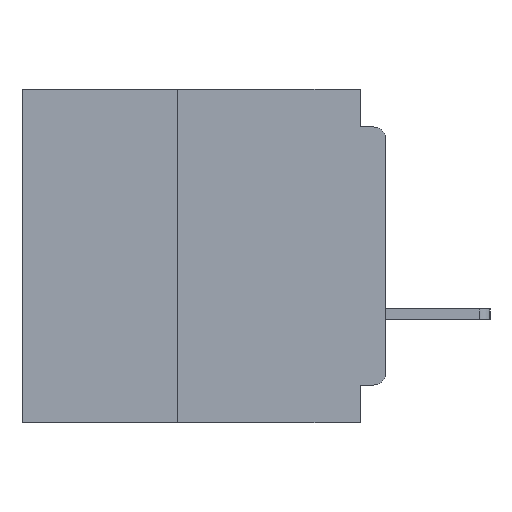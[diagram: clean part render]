
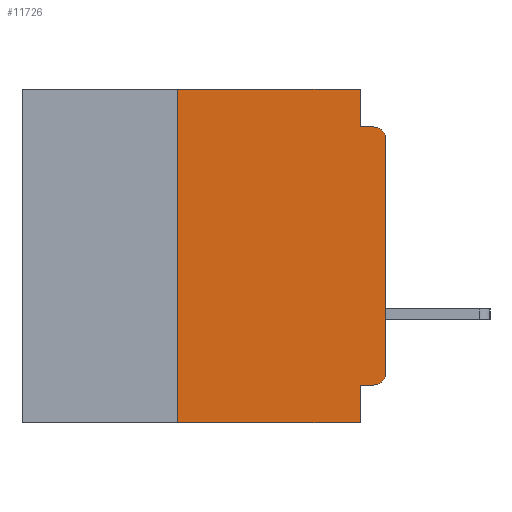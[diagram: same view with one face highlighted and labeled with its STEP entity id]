
A CAD part, left-side view. The second image highlights one B-rep face of the part: STEP entity #11726.
In plain terms, the highlighted planar face has unit normal (-1, 0, 0).
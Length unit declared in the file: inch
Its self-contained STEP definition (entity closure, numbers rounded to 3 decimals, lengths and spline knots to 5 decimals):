
#1133 = EDGE_CURVE ( 'NONE', #33137, #47126, #41011, .T. ) ;
#1188 = VECTOR ( 'NONE', #29116, 39.37008 ) ;
#1340 = CIRCLE ( 'NONE', #21619, 0.015 ) ;
#1385 = ORIENTED_EDGE ( 'NONE', *, *, #33223, .T. ) ;
#3551 = EDGE_CURVE ( 'NONE', #46628, #23718, #9136, .T. ) ;
#3782 = EDGE_CURVE ( 'NONE', #47126, #16703, #18458, .T. ) ;
#3885 = PLANE ( 'NONE',  #14189 ) ;
#4304 = LINE ( 'NONE', #25368, #42964 ) ;
#5230 = EDGE_CURVE ( 'NONE', #31758, #46628, #37131, .T. ) ;
#6052 = LINE ( 'NONE', #44029, #17165 ) ;
#7671 = CARTESIAN_POINT ( 'NONE',  ( 0., 0.437, 0. ) ) ;
#8571 = ORIENTED_EDGE ( 'NONE', *, *, #3782, .F. ) ;
#8986 = FACE_OUTER_BOUND ( 'NONE', #24166, .T. ) ;
#9136 = LINE ( 'NONE', #38466, #37839 ) ;
#11415 = DIRECTION ( 'NONE',  ( 0., 0., -1. ) ) ;
#11451 = ORIENTED_EDGE ( 'NONE', *, *, #3551, .F. ) ;
#11491 = CARTESIAN_POINT ( 'NONE',  ( 0., 0.25, 0. ) ) ;
#11572 = EDGE_CURVE ( 'NONE', #14571, #30251, #6052, .T. ) ;
#11726 = ADVANCED_FACE ( 'NONE', ( #8986 ), #3885, .F. ) ;
#13994 = CARTESIAN_POINT ( 'NONE',  ( 0., 0.015, -0.355 ) ) ;
#14189 = AXIS2_PLACEMENT_3D ( 'NONE', #7671, #33876, #11415 ) ;
#14262 = EDGE_CURVE ( 'NONE', #33137, #14571, #38580, .T. ) ;
#14571 = VERTEX_POINT ( 'NONE', #34019 ) ;
#16144 = DIRECTION ( 'NONE',  ( -1., 0., 0. ) ) ;
#16207 = VECTOR ( 'NONE', #44451, 39.37008 ) ;
#16296 = ORIENTED_EDGE ( 'NONE', *, *, #5230, .F. ) ;
#16703 = VERTEX_POINT ( 'NONE', #31825 ) ;
#17165 = VECTOR ( 'NONE', #32747, 39.37008 ) ;
#17273 = VECTOR ( 'NONE', #23125, 39.37008 ) ;
#18458 = LINE ( 'NONE', #23476, #17273 ) ;
#19808 = ORIENTED_EDGE ( 'NONE', *, *, #29904, .F. ) ;
#19829 = LINE ( 'NONE', #27886, #38569 ) ;
#21082 = CARTESIAN_POINT ( 'NONE',  ( 0., 0.015, -0.34 ) ) ;
#21416 = VERTEX_POINT ( 'NONE', #11491 ) ;
#21619 = AXIS2_PLACEMENT_3D ( 'NONE', #38604, #16144, #42370 ) ;
#23125 = DIRECTION ( 'NONE',  ( 0., 0., -1. ) ) ;
#23476 = CARTESIAN_POINT ( 'NONE',  ( 0., 0.031, -0.4 ) ) ;
#23643 = DIRECTION ( 'NONE',  ( 0., 0., -1. ) ) ;
#23718 = VERTEX_POINT ( 'NONE', #42713 ) ;
#23805 = CARTESIAN_POINT ( 'NONE',  ( 0., 0.031, 0. ) ) ;
#24166 = EDGE_LOOP ( 'NONE', ( #44445, #28306, #11451, #16296, #19808, #26790, #1385, #8571, #32576, #24801 ) ) ;
#24236 = DIRECTION ( 'NONE',  ( 0., 0., 1. ) ) ;
#24801 = ORIENTED_EDGE ( 'NONE', *, *, #14262, .T. ) ;
#24826 = DIRECTION ( 'NONE',  ( 0., 0., -1. ) ) ;
#25368 = CARTESIAN_POINT ( 'NONE',  ( 0., 0.437, 0. ) ) ;
#26790 = ORIENTED_EDGE ( 'NONE', *, *, #39992, .F. ) ;
#27885 = VERTEX_POINT ( 'NONE', #46552 ) ;
#27886 = CARTESIAN_POINT ( 'NONE',  ( 0., 0.25, -0.4 ) ) ;
#28306 = ORIENTED_EDGE ( 'NONE', *, *, #30213, .T. ) ;
#29116 = DIRECTION ( 'NONE',  ( 0., 1., 0. ) ) ;
#29137 = AXIS2_PLACEMENT_3D ( 'NONE', #21082, #47265, #24826 ) ;
#29191 = DIRECTION ( 'NONE',  ( 0., -1., 0. ) ) ;
#29242 = CARTESIAN_POINT ( 'NONE',  ( 0., 0., -0.355 ) ) ;
#29904 = EDGE_CURVE ( 'NONE', #21416, #31758, #4304, .T. ) ;
#30213 = EDGE_CURVE ( 'NONE', #30251, #23718, #1340, .T. ) ;
#30251 = VERTEX_POINT ( 'NONE', #46296 ) ;
#31758 = VERTEX_POINT ( 'NONE', #44859 ) ;
#31825 = CARTESIAN_POINT ( 'NONE',  ( 0., 0.031, -0.4 ) ) ;
#32576 = ORIENTED_EDGE ( 'NONE', *, *, #1133, .F. ) ;
#32747 = DIRECTION ( 'NONE',  ( 0., 0., 1. ) ) ;
#33137 = VERTEX_POINT ( 'NONE', #13994 ) ;
#33223 = EDGE_CURVE ( 'NONE', #27885, #16703, #46121, .T. ) ;
#33876 = DIRECTION ( 'NONE',  ( 1., 0., 0. ) ) ;
#34019 = CARTESIAN_POINT ( 'NONE',  ( 0., 0., -0.34 ) ) ;
#35799 = CARTESIAN_POINT ( 'NONE',  ( 0., 0.031, -0.355 ) ) ;
#36925 = CARTESIAN_POINT ( 'NONE',  ( 0., 0.437, -0.4 ) ) ;
#37131 = LINE ( 'NONE', #23805, #45909 ) ;
#37839 = VECTOR ( 'NONE', #38558, 39.37008 ) ;
#38466 = CARTESIAN_POINT ( 'NONE',  ( 0., 0., -0.045 ) ) ;
#38558 = DIRECTION ( 'NONE',  ( 0., -1., 0. ) ) ;
#38569 = VECTOR ( 'NONE', #24236, 39.37008 ) ;
#38580 = CIRCLE ( 'NONE', #29137, 0.015 ) ;
#38604 = CARTESIAN_POINT ( 'NONE',  ( 0., 0.015, -0.06 ) ) ;
#39992 = EDGE_CURVE ( 'NONE', #27885, #21416, #19829, .T. ) ;
#40081 = CARTESIAN_POINT ( 'NONE',  ( 0., 0.031, -0.045 ) ) ;
#41011 = LINE ( 'NONE', #29242, #1188 ) ;
#42370 = DIRECTION ( 'NONE',  ( 0., 0., -1. ) ) ;
#42713 = CARTESIAN_POINT ( 'NONE',  ( 0., 0.015, -0.045 ) ) ;
#42964 = VECTOR ( 'NONE', #29191, 39.37008 ) ;
#44029 = CARTESIAN_POINT ( 'NONE',  ( 0., 0., 0. ) ) ;
#44445 = ORIENTED_EDGE ( 'NONE', *, *, #11572, .T. ) ;
#44451 = DIRECTION ( 'NONE',  ( 0., -1., 0. ) ) ;
#44859 = CARTESIAN_POINT ( 'NONE',  ( 0., 0.031, 0. ) ) ;
#45909 = VECTOR ( 'NONE', #23643, 39.37008 ) ;
#46121 = LINE ( 'NONE', #36925, #16207 ) ;
#46296 = CARTESIAN_POINT ( 'NONE',  ( 0., 0., -0.06 ) ) ;
#46552 = CARTESIAN_POINT ( 'NONE',  ( 0., 0.25, -0.4 ) ) ;
#46628 = VERTEX_POINT ( 'NONE', #40081 ) ;
#47126 = VERTEX_POINT ( 'NONE', #35799 ) ;
#47265 = DIRECTION ( 'NONE',  ( -1., 0., 0. ) ) ;
